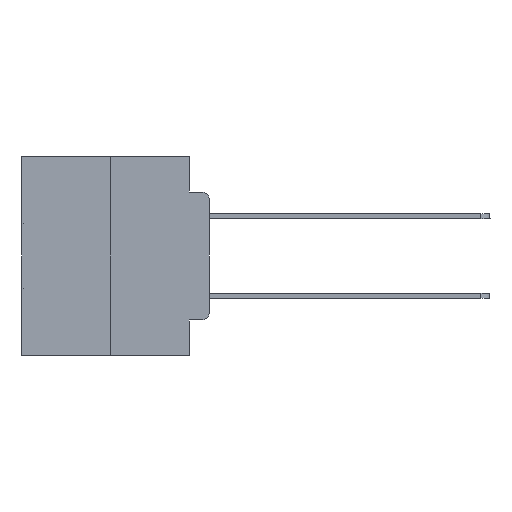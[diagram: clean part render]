
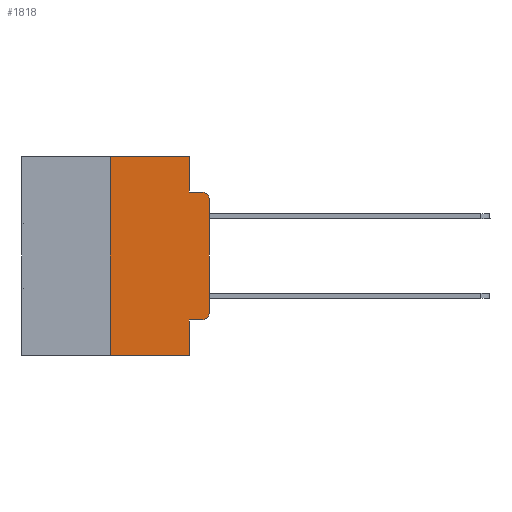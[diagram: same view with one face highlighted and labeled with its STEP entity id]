
A CAD part, left-side view. The second image highlights one B-rep face of the part: STEP entity #1818.
In plain terms, the highlighted planar face has unit normal (-1, 0, 0).
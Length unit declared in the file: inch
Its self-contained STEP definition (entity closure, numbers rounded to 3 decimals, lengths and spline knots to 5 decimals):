
#742 = CARTESIAN_POINT ( 'NONE',  ( 0., 0.02, -0.3915 ) ) ;
#787 = VECTOR ( 'NONE', #20521, 39.37008 ) ;
#1658 = VERTEX_POINT ( 'NONE', #30008 ) ;
#1818 = ADVANCED_FACE ( 'NONE', ( #23914 ), #19164, .F. ) ;
#2116 = VERTEX_POINT ( 'NONE', #15111 ) ;
#2601 = ORIENTED_EDGE ( 'NONE', *, *, #24910, .T. ) ;
#2727 = VECTOR ( 'NONE', #16096, 39.37008 ) ;
#3248 = VERTEX_POINT ( 'NONE', #3544 ) ;
#3544 = CARTESIAN_POINT ( 'NONE',  ( 0., 0.02, -0.0885 ) ) ;
#4357 = EDGE_CURVE ( 'NONE', #21248, #3248, #4570, .T. ) ;
#4570 = LINE ( 'NONE', #9074, #10187 ) ;
#5174 = EDGE_CURVE ( 'NONE', #2116, #11791, #11655, .T. ) ;
#6392 = CARTESIAN_POINT ( 'NONE',  ( 0., 0.051, 0. ) ) ;
#6542 = ORIENTED_EDGE ( 'NONE', *, *, #4357, .F. ) ;
#7149 = CARTESIAN_POINT ( 'NONE',  ( 0., 0.051, -0.4115 ) ) ;
#7243 = LINE ( 'NONE', #26226, #29525 ) ;
#7313 = CARTESIAN_POINT ( 'NONE',  ( 0., 0.473, -0.5 ) ) ;
#7314 = ORIENTED_EDGE ( 'NONE', *, *, #20597, .T. ) ;
#7469 = DIRECTION ( 'NONE',  ( -1., 0., 0. ) ) ;
#7525 = VECTOR ( 'NONE', #15802, 39.37008 ) ;
#8280 = EDGE_CURVE ( 'NONE', #26879, #21248, #16284, .T. ) ;
#8417 = CARTESIAN_POINT ( 'NONE',  ( 0., 0.051, 0. ) ) ;
#9074 = CARTESIAN_POINT ( 'NONE',  ( 0., 0.051, -0.0885 ) ) ;
#9292 = DIRECTION ( 'NONE',  ( 0., -1., 0. ) ) ;
#9597 = ORIENTED_EDGE ( 'NONE', *, *, #17646, .F. ) ;
#10078 = LINE ( 'NONE', #7313, #20252 ) ;
#10127 = VECTOR ( 'NONE', #26433, 39.37008 ) ;
#10187 = VECTOR ( 'NONE', #9292, 39.37008 ) ;
#10610 = CARTESIAN_POINT ( 'NONE',  ( 0., 0.25, 0. ) ) ;
#10702 = AXIS2_PLACEMENT_3D ( 'NONE', #21558, #11652, #14411 ) ;
#11260 = EDGE_CURVE ( 'NONE', #11791, #29082, #17984, .T. ) ;
#11652 = DIRECTION ( 'NONE',  ( 1., 0., 0. ) ) ;
#11655 = LINE ( 'NONE', #7149, #10127 ) ;
#11791 = VERTEX_POINT ( 'NONE', #29368 ) ;
#12726 = CARTESIAN_POINT ( 'NONE',  ( 0., 0.25, -0.5 ) ) ;
#13576 = ORIENTED_EDGE ( 'NONE', *, *, #8280, .F. ) ;
#13970 = ORIENTED_EDGE ( 'NONE', *, *, #5174, .T. ) ;
#14411 = DIRECTION ( 'NONE',  ( 0., 0., -1. ) ) ;
#14952 = ORIENTED_EDGE ( 'NONE', *, *, #15149, .F. ) ;
#15111 = CARTESIAN_POINT ( 'NONE',  ( 0., 0.051, -0.4115 ) ) ;
#15149 = EDGE_CURVE ( 'NONE', #1658, #26879, #20112, .T. ) ;
#15802 = DIRECTION ( 'NONE',  ( 0., 0., -1. ) ) ;
#16096 = DIRECTION ( 'NONE',  ( 0., 0., -1. ) ) ;
#16284 = LINE ( 'NONE', #6392, #2727 ) ;
#16370 = ORIENTED_EDGE ( 'NONE', *, *, #11260, .T. ) ;
#16728 = DIRECTION ( 'NONE',  ( 0., 0., 1. ) ) ;
#16908 = EDGE_LOOP ( 'NONE', ( #24357, #7314, #6542, #13576, #14952, #9597, #2601, #19489, #13970, #16370 ) ) ;
#17188 = DIRECTION ( 'NONE',  ( 0., 0., -1. ) ) ;
#17368 = LINE ( 'NONE', #10610, #787 ) ;
#17484 = VECTOR ( 'NONE', #22744, 39.37008 ) ;
#17511 = VERTEX_POINT ( 'NONE', #17694 ) ;
#17646 = EDGE_CURVE ( 'NONE', #24541, #1658, #17368, .T. ) ;
#17694 = CARTESIAN_POINT ( 'NONE',  ( 0., 0.051, -0.5 ) ) ;
#17732 = LINE ( 'NONE', #8417, #7525 ) ;
#17984 = CIRCLE ( 'NONE', #30874, 0.02 ) ;
#18896 = CARTESIAN_POINT ( 'NONE',  ( 0., 0.051, -0.0885 ) ) ;
#19164 = PLANE ( 'NONE',  #10702 ) ;
#19433 = CIRCLE ( 'NONE', #27858, 0.02 ) ;
#19489 = ORIENTED_EDGE ( 'NONE', *, *, #23722, .F. ) ;
#20112 = LINE ( 'NONE', #29941, #17484 ) ;
#20252 = VECTOR ( 'NONE', #21749, 39.37008 ) ;
#20297 = CARTESIAN_POINT ( 'NONE',  ( 0., 0., -0.1085 ) ) ;
#20400 = DIRECTION ( 'NONE',  ( -1., 0., 0. ) ) ;
#20521 = DIRECTION ( 'NONE',  ( 0., 0., 1. ) ) ;
#20597 = EDGE_CURVE ( 'NONE', #24288, #3248, #19433, .T. ) ;
#21148 = CARTESIAN_POINT ( 'NONE',  ( 0., 0., -0.3915 ) ) ;
#21248 = VERTEX_POINT ( 'NONE', #18896 ) ;
#21558 = CARTESIAN_POINT ( 'NONE',  ( 0., 0.473, 0. ) ) ;
#21749 = DIRECTION ( 'NONE',  ( 0., -1., 0. ) ) ;
#22744 = DIRECTION ( 'NONE',  ( 0., -1., 0. ) ) ;
#23722 = EDGE_CURVE ( 'NONE', #2116, #17511, #17732, .T. ) ;
#23914 = FACE_OUTER_BOUND ( 'NONE', #16908, .T. ) ;
#24288 = VERTEX_POINT ( 'NONE', #20297 ) ;
#24357 = ORIENTED_EDGE ( 'NONE', *, *, #30299, .T. ) ;
#24541 = VERTEX_POINT ( 'NONE', #12726 ) ;
#24910 = EDGE_CURVE ( 'NONE', #24541, #17511, #10078, .T. ) ;
#26226 = CARTESIAN_POINT ( 'NONE',  ( 0., 0., 0. ) ) ;
#26433 = DIRECTION ( 'NONE',  ( 0., -1., 0. ) ) ;
#26608 = CARTESIAN_POINT ( 'NONE',  ( 0., 0.051, 0. ) ) ;
#26879 = VERTEX_POINT ( 'NONE', #26608 ) ;
#27858 = AXIS2_PLACEMENT_3D ( 'NONE', #29414, #7469, #17188 ) ;
#29082 = VERTEX_POINT ( 'NONE', #21148 ) ;
#29368 = CARTESIAN_POINT ( 'NONE',  ( 0., 0.02, -0.4115 ) ) ;
#29414 = CARTESIAN_POINT ( 'NONE',  ( 0., 0.02, -0.1085 ) ) ;
#29525 = VECTOR ( 'NONE', #16728, 39.37008 ) ;
#29805 = DIRECTION ( 'NONE',  ( 0., 0., -1. ) ) ;
#29941 = CARTESIAN_POINT ( 'NONE',  ( 0., 0.473, 0. ) ) ;
#30008 = CARTESIAN_POINT ( 'NONE',  ( 0., 0.25, 0. ) ) ;
#30299 = EDGE_CURVE ( 'NONE', #29082, #24288, #7243, .T. ) ;
#30874 = AXIS2_PLACEMENT_3D ( 'NONE', #742, #20400, #29805 ) ;
